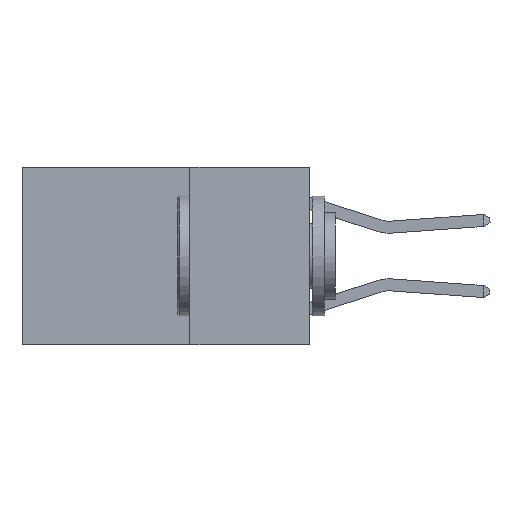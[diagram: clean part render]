
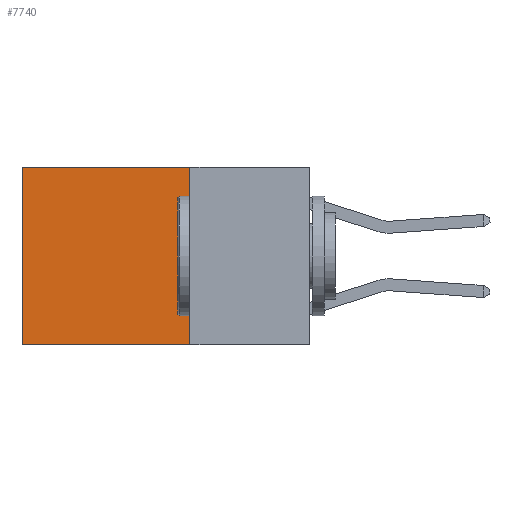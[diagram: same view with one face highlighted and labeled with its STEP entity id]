
A CAD part, left-side view. The second image highlights one B-rep face of the part: STEP entity #7740.
In plain terms, the highlighted planar face has unit normal (-1, 0, 0).
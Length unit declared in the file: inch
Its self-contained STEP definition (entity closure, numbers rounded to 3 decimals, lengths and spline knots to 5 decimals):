
#14 = VECTOR ( 'NONE', #8793, 39.37008 ) ;
#150 = LINE ( 'NONE', #6228, #8116 ) ;
#407 = ORIENTED_EDGE ( 'NONE', *, *, #1243, .F. ) ;
#548 = VECTOR ( 'NONE', #9956, 39.37008 ) ;
#854 = AXIS2_PLACEMENT_3D ( 'NONE', #3692, #7407, #2946 ) ;
#1243 = EDGE_CURVE ( 'NONE', #3404, #4036, #150, .T. ) ;
#1358 = PLANE ( 'NONE',  #854 ) ;
#1367 = LINE ( 'NONE', #3422, #14 ) ;
#1607 = DIRECTION ( 'NONE',  ( 0., 0., -1. ) ) ;
#1886 = VERTEX_POINT ( 'NONE', #3092 ) ;
#2007 = CARTESIAN_POINT ( 'NONE',  ( 0.2625, 0.6, -0.37 ) ) ;
#2014 = CARTESIAN_POINT ( 'NONE',  ( 0.2625, 0.25, -0.37 ) ) ;
#2759 = VERTEX_POINT ( 'NONE', #2007 ) ;
#2946 = DIRECTION ( 'NONE',  ( 0., 0., -1. ) ) ;
#3092 = CARTESIAN_POINT ( 'NONE',  ( 0.2625, 0.6, 0. ) ) ;
#3404 = VERTEX_POINT ( 'NONE', #4864 ) ;
#3422 = CARTESIAN_POINT ( 'NONE',  ( 0.2625, 0.6, 0. ) ) ;
#3692 = CARTESIAN_POINT ( 'NONE',  ( 0.2625, 0.25, 0. ) ) ;
#3779 = CARTESIAN_POINT ( 'NONE',  ( 0.2625, 0.25, -0.37 ) ) ;
#4036 = VERTEX_POINT ( 'NONE', #3779 ) ;
#4280 = VECTOR ( 'NONE', #9809, 39.37008 ) ;
#4615 = EDGE_LOOP ( 'NONE', ( #8196, #8420, #407, #5219 ) ) ;
#4864 = CARTESIAN_POINT ( 'NONE',  ( 0.2625, 0.25, 0. ) ) ;
#5219 = ORIENTED_EDGE ( 'NONE', *, *, #6118, .T. ) ;
#5297 = CARTESIAN_POINT ( 'NONE',  ( 0.2625, 0.25, 0. ) ) ;
#6118 = EDGE_CURVE ( 'NONE', #3404, #1886, #8010, .T. ) ;
#6228 = CARTESIAN_POINT ( 'NONE',  ( 0.2625, 0.25, 0. ) ) ;
#6411 = FACE_OUTER_BOUND ( 'NONE', #4615, .T. ) ;
#6539 = LINE ( 'NONE', #2014, #4280 ) ;
#7238 = EDGE_CURVE ( 'NONE', #1886, #2759, #1367, .T. ) ;
#7382 = EDGE_CURVE ( 'NONE', #4036, #2759, #6539, .T. ) ;
#7407 = DIRECTION ( 'NONE',  ( 1., 0., 0. ) ) ;
#7740 = ADVANCED_FACE ( 'NONE', ( #6411 ), #1358, .F. ) ;
#8010 = LINE ( 'NONE', #5297, #548 ) ;
#8116 = VECTOR ( 'NONE', #1607, 39.37008 ) ;
#8196 = ORIENTED_EDGE ( 'NONE', *, *, #7238, .T. ) ;
#8420 = ORIENTED_EDGE ( 'NONE', *, *, #7382, .F. ) ;
#8793 = DIRECTION ( 'NONE',  ( 0., 0., -1. ) ) ;
#9809 = DIRECTION ( 'NONE',  ( 0., 1., 0. ) ) ;
#9956 = DIRECTION ( 'NONE',  ( 0., 1., 0. ) ) ;
